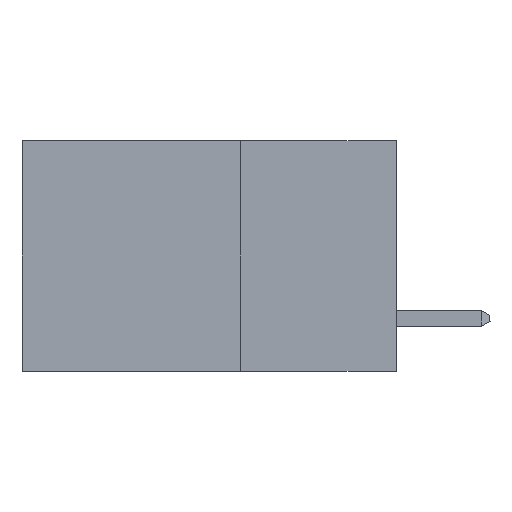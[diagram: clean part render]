
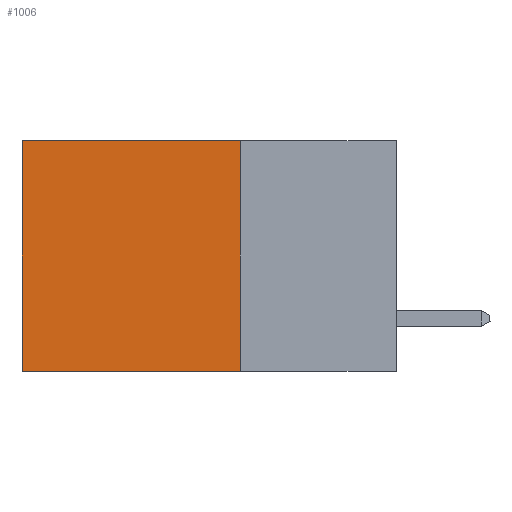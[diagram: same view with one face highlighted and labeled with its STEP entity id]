
A CAD part, left-side view. The second image highlights one B-rep face of the part: STEP entity #1006.
In plain terms, the highlighted planar face has unit normal (-1, 0, 0).
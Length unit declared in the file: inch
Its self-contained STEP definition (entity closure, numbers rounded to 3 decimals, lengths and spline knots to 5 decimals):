
#1006 = ADVANCED_FACE ( 'NONE', ( #3820 ), #4292, .F. ) ;
#1748 = CARTESIAN_POINT ( 'NONE',  ( 0.298, 0.25, 0. ) ) ;
#3820 = FACE_OUTER_BOUND ( 'NONE', #15046, .T. ) ;
#3876 = VERTEX_POINT ( 'NONE', #8982 ) ;
#4292 = PLANE ( 'NONE',  #11438 ) ;
#4808 = EDGE_CURVE ( 'NONE', #5114, #19962, #11050, .T. ) ;
#5114 = VERTEX_POINT ( 'NONE', #1748 ) ;
#5431 = CARTESIAN_POINT ( 'NONE',  ( 0.298, 0.6, -0.37 ) ) ;
#7509 = EDGE_CURVE ( 'NONE', #19962, #13490, #21549, .T. ) ;
#7551 = EDGE_CURVE ( 'NONE', #3876, #13490, #12827, .T. ) ;
#7605 = VECTOR ( 'NONE', #9502, 39.37008 ) ;
#7772 = CARTESIAN_POINT ( 'NONE',  ( 0.298, 0.25, 0. ) ) ;
#8537 = ORIENTED_EDGE ( 'NONE', *, *, #4808, .T. ) ;
#8839 = ORIENTED_EDGE ( 'NONE', *, *, #7509, .T. ) ;
#8982 = CARTESIAN_POINT ( 'NONE',  ( 0.298, 0.25, -0.37 ) ) ;
#9502 = DIRECTION ( 'NONE',  ( 0., 1., 0. ) ) ;
#10060 = ORIENTED_EDGE ( 'NONE', *, *, #7551, .F. ) ;
#10368 = EDGE_CURVE ( 'NONE', #5114, #3876, #19906, .T. ) ;
#10439 = CARTESIAN_POINT ( 'NONE',  ( 0.298, 0.25, 0. ) ) ;
#11050 = LINE ( 'NONE', #10439, #14545 ) ;
#11438 = AXIS2_PLACEMENT_3D ( 'NONE', #7772, #21628, #18005 ) ;
#12827 = LINE ( 'NONE', #13096, #7605 ) ;
#12927 = DIRECTION ( 'NONE',  ( 0., 0., -1. ) ) ;
#13053 = CARTESIAN_POINT ( 'NONE',  ( 0.298, 0.25, 0. ) ) ;
#13096 = CARTESIAN_POINT ( 'NONE',  ( 0.298, 0.25, -0.37 ) ) ;
#13490 = VERTEX_POINT ( 'NONE', #5431 ) ;
#13818 = DIRECTION ( 'NONE',  ( 0., 0., -1. ) ) ;
#14008 = CARTESIAN_POINT ( 'NONE',  ( 0.298, 0.6, 0. ) ) ;
#14545 = VECTOR ( 'NONE', #18952, 39.37008 ) ;
#15046 = EDGE_LOOP ( 'NONE', ( #8839, #10060, #15412, #8537 ) ) ;
#15056 = VECTOR ( 'NONE', #12927, 39.37008 ) ;
#15412 = ORIENTED_EDGE ( 'NONE', *, *, #10368, .F. ) ;
#17181 = VECTOR ( 'NONE', #13818, 39.37008 ) ;
#18005 = DIRECTION ( 'NONE',  ( 0., 0., -1. ) ) ;
#18952 = DIRECTION ( 'NONE',  ( 0., 1., 0. ) ) ;
#19906 = LINE ( 'NONE', #13053, #15056 ) ;
#19962 = VERTEX_POINT ( 'NONE', #21271 ) ;
#21271 = CARTESIAN_POINT ( 'NONE',  ( 0.298, 0.6, 0. ) ) ;
#21549 = LINE ( 'NONE', #14008, #17181 ) ;
#21628 = DIRECTION ( 'NONE',  ( 1., 0., 0. ) ) ;
